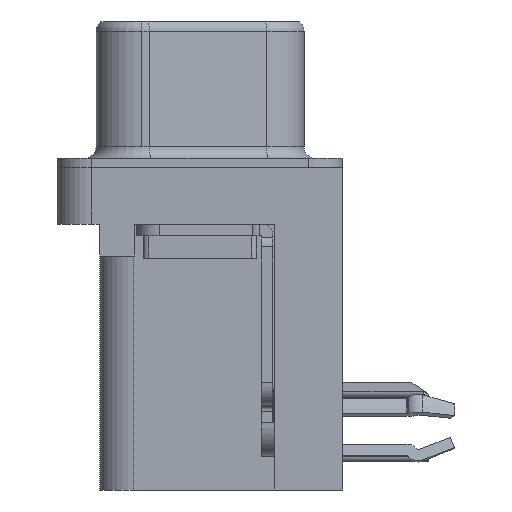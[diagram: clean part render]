
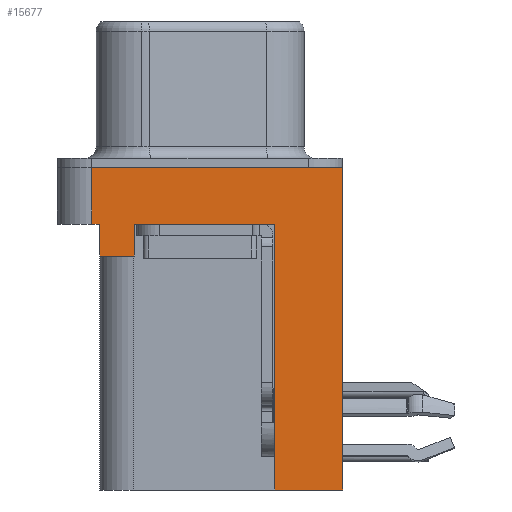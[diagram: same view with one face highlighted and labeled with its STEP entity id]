
A CAD part, left-side view. The second image highlights one B-rep face of the part: STEP entity #15677.
In plain terms, the highlighted planar face has unit normal (-1, 0, 0).
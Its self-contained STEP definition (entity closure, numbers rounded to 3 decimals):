
#347 = VECTOR ( 'NONE', #15084, 1000. ) ;
#586 = VERTEX_POINT ( 'NONE', #12006 ) ;
#601 = DIRECTION ( 'NONE',  ( 0., 0., 1. ) ) ;
#666 = EDGE_CURVE ( 'NONE', #16573, #669, #7526, .T. ) ;
#669 = VERTEX_POINT ( 'NONE', #4343 ) ;
#841 = DIRECTION ( 'NONE',  ( 0., 0., 1. ) ) ;
#1040 = ORIENTED_EDGE ( 'NONE', *, *, #2394, .T. ) ;
#1182 = ORIENTED_EDGE ( 'NONE', *, *, #11094, .F. ) ;
#1481 = CARTESIAN_POINT ( 'NONE',  ( -2.91, 4.425, -3.9 ) ) ;
#1617 = CARTESIAN_POINT ( 'NONE',  ( -2.91, 4.425, -3.9 ) ) ;
#1758 = VERTEX_POINT ( 'NONE', #1481 ) ;
#2255 = CARTESIAN_POINT ( 'NONE',  ( -2.91, -6.275, -2.5 ) ) ;
#2345 = VERTEX_POINT ( 'NONE', #8211 ) ;
#2394 = EDGE_CURVE ( 'NONE', #8325, #12197, #4368, .T. ) ;
#2500 = ORIENTED_EDGE ( 'NONE', *, *, #9090, .F. ) ;
#2809 = CARTESIAN_POINT ( 'NONE',  ( -2.91, -3.295, -2.5 ) ) ;
#2869 = DIRECTION ( 'NONE',  ( 0., -1., 0. ) ) ;
#3027 = DIRECTION ( 'NONE',  ( 0., 0., 1. ) ) ;
#3203 = VECTOR ( 'NONE', #15233, 1000. ) ;
#3296 = VECTOR ( 'NONE', #17002, 1000. ) ;
#3366 = DIRECTION ( 'NONE',  ( 0., -1., 0. ) ) ;
#3537 = EDGE_CURVE ( 'NONE', #586, #2345, #13031, .T. ) ;
#3926 = LINE ( 'NONE', #5119, #347 ) ;
#4343 = CARTESIAN_POINT ( 'NONE',  ( -2.91, -6.275, 0. ) ) ;
#4368 = LINE ( 'NONE', #16630, #16508 ) ;
#4986 = DIRECTION ( 'NONE',  ( 0., 0., 1. ) ) ;
#5119 = CARTESIAN_POINT ( 'NONE',  ( -2.91, -3.295, -14.2 ) ) ;
#5159 = VECTOR ( 'NONE', #3366, 1000. ) ;
#5472 = VECTOR ( 'NONE', #601, 1000. ) ;
#5762 = CARTESIAN_POINT ( 'NONE',  ( -2.91, -6.275, 0. ) ) ;
#5819 = AXIS2_PLACEMENT_3D ( 'NONE', #2255, #13018, #4986 ) ;
#5844 = CARTESIAN_POINT ( 'NONE',  ( -2.91, 2.895, -2.5 ) ) ;
#6021 = LINE ( 'NONE', #5762, #17874 ) ;
#6082 = PLANE ( 'NONE',  #5819 ) ;
#6890 = CARTESIAN_POINT ( 'NONE',  ( -2.91, 4.425, -3.9 ) ) ;
#7058 = EDGE_CURVE ( 'NONE', #8046, #15881, #8131, .T. ) ;
#7082 = EDGE_CURVE ( 'NONE', #16573, #8046, #3926, .T. ) ;
#7088 = DIRECTION ( 'NONE',  ( 0., 0., 1. ) ) ;
#7445 = FACE_OUTER_BOUND ( 'NONE', #12651, .T. ) ;
#7526 = LINE ( 'NONE', #13098, #5472 ) ;
#7612 = EDGE_CURVE ( 'NONE', #586, #11015, #13256, .T. ) ;
#7678 = CARTESIAN_POINT ( 'NONE',  ( -2.91, -6.275, -14.2 ) ) ;
#7827 = ORIENTED_EDGE ( 'NONE', *, *, #9627, .T. ) ;
#8046 = VERTEX_POINT ( 'NONE', #17888 ) ;
#8131 = LINE ( 'NONE', #15179, #10547 ) ;
#8192 = ORIENTED_EDGE ( 'NONE', *, *, #666, .T. ) ;
#8202 = ORIENTED_EDGE ( 'NONE', *, *, #7612, .F. ) ;
#8211 = CARTESIAN_POINT ( 'NONE',  ( -2.91, 4.425, -2.5 ) ) ;
#8325 = VERTEX_POINT ( 'NONE', #10190 ) ;
#8363 = CARTESIAN_POINT ( 'NONE',  ( -2.91, 4.775, 0. ) ) ;
#8461 = LINE ( 'NONE', #1617, #14973 ) ;
#9090 = EDGE_CURVE ( 'NONE', #11015, #669, #6021, .T. ) ;
#9134 = ORIENTED_EDGE ( 'NONE', *, *, #7058, .F. ) ;
#9627 = EDGE_CURVE ( 'NONE', #12197, #15881, #13972, .T. ) ;
#10190 = CARTESIAN_POINT ( 'NONE',  ( -2.91, 2.895, -3.9 ) ) ;
#10547 = VECTOR ( 'NONE', #16192, 1000. ) ;
#10836 = LINE ( 'NONE', #6890, #3203 ) ;
#10875 = VECTOR ( 'NONE', #841, 1000. ) ;
#11015 = VERTEX_POINT ( 'NONE', #8363 ) ;
#11094 = EDGE_CURVE ( 'NONE', #1758, #2345, #8461, .T. ) ;
#11218 = ORIENTED_EDGE ( 'NONE', *, *, #3537, .T. ) ;
#11542 = ORIENTED_EDGE ( 'NONE', *, *, #15834, .F. ) ;
#12006 = CARTESIAN_POINT ( 'NONE',  ( -2.91, 4.775, -2.5 ) ) ;
#12197 = VERTEX_POINT ( 'NONE', #5844 ) ;
#12651 = EDGE_LOOP ( 'NONE', ( #2500, #8202, #11218, #1182, #11542, #1040, #7827, #9134, #14294, #8192 ) ) ;
#13018 = DIRECTION ( 'NONE',  ( -1., 0., 0. ) ) ;
#13031 = LINE ( 'NONE', #14330, #5159 ) ;
#13098 = CARTESIAN_POINT ( 'NONE',  ( -2.91, -6.275, -2.5 ) ) ;
#13256 = LINE ( 'NONE', #14736, #10875 ) ;
#13972 = LINE ( 'NONE', #17333, #3296 ) ;
#14294 = ORIENTED_EDGE ( 'NONE', *, *, #7082, .F. ) ;
#14330 = CARTESIAN_POINT ( 'NONE',  ( -2.91, -6.275, -2.5 ) ) ;
#14736 = CARTESIAN_POINT ( 'NONE',  ( -2.91, 4.775, -2.5 ) ) ;
#14973 = VECTOR ( 'NONE', #7088, 1000. ) ;
#15084 = DIRECTION ( 'NONE',  ( 0., 1., 0. ) ) ;
#15179 = CARTESIAN_POINT ( 'NONE',  ( -2.91, -3.295, -14.2 ) ) ;
#15233 = DIRECTION ( 'NONE',  ( 0., 1., 0. ) ) ;
#15677 = ADVANCED_FACE ( 'NONE', ( #7445 ), #6082, .T. ) ;
#15834 = EDGE_CURVE ( 'NONE', #8325, #1758, #10836, .T. ) ;
#15881 = VERTEX_POINT ( 'NONE', #2809 ) ;
#16192 = DIRECTION ( 'NONE',  ( 0., 0., 1. ) ) ;
#16508 = VECTOR ( 'NONE', #3027, 1000. ) ;
#16573 = VERTEX_POINT ( 'NONE', #7678 ) ;
#16630 = CARTESIAN_POINT ( 'NONE',  ( -2.91, 2.895, -3.9 ) ) ;
#17002 = DIRECTION ( 'NONE',  ( 0., -1., 0. ) ) ;
#17333 = CARTESIAN_POINT ( 'NONE',  ( -2.91, -6.275, -2.5 ) ) ;
#17874 = VECTOR ( 'NONE', #2869, 1000. ) ;
#17888 = CARTESIAN_POINT ( 'NONE',  ( -2.91, -3.295, -14.2 ) ) ;
